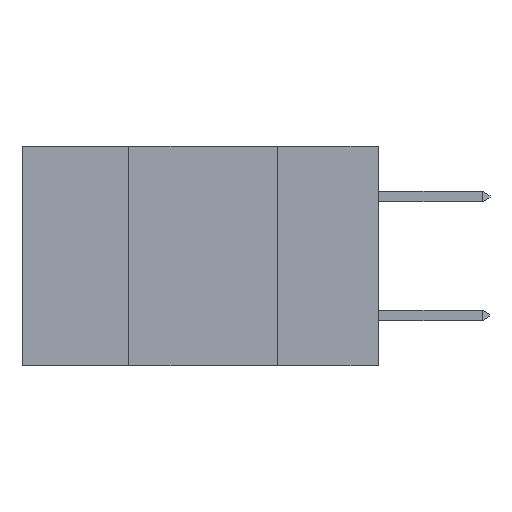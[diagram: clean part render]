
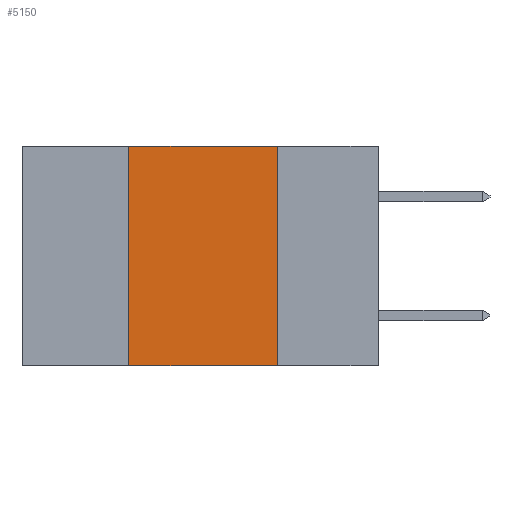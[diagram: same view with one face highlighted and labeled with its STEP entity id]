
A CAD part, left-side view. The second image highlights one B-rep face of the part: STEP entity #5150.
In plain terms, the highlighted planar face has unit normal (-1, 0, 0).
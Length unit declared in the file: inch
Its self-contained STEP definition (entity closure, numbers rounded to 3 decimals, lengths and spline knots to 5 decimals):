
#584 = ORIENTED_EDGE ( 'NONE', *, *, #10975, .F. ) ;
#1240 = VERTEX_POINT ( 'NONE', #1879 ) ;
#1879 = CARTESIAN_POINT ( 'NONE',  ( 0., 0.17, -0.37 ) ) ;
#2287 = DIRECTION ( 'NONE',  ( 0., 0., -1. ) ) ;
#2360 = VECTOR ( 'NONE', #20939, 39.37008 ) ;
#2624 = DIRECTION ( 'NONE',  ( 0., 0., 1. ) ) ;
#2678 = LINE ( 'NONE', #19572, #13314 ) ;
#2718 = ORIENTED_EDGE ( 'NONE', *, *, #19163, .F. ) ;
#2995 = CARTESIAN_POINT ( 'NONE',  ( 0., 0.42, -0.37 ) ) ;
#4079 = EDGE_CURVE ( 'NONE', #15891, #11140, #4483, .T. ) ;
#4483 = LINE ( 'NONE', #10596, #13944 ) ;
#5150 = ADVANCED_FACE ( 'NONE', ( #6834 ), #5991, .F. ) ;
#5981 = ORIENTED_EDGE ( 'NONE', *, *, #4079, .F. ) ;
#5991 = PLANE ( 'NONE',  #22442 ) ;
#6834 = FACE_OUTER_BOUND ( 'NONE', #9041, .T. ) ;
#7362 = LINE ( 'NONE', #9737, #2360 ) ;
#7534 = CARTESIAN_POINT ( 'NONE',  ( 0., 0.6, -0.37 ) ) ;
#9041 = EDGE_LOOP ( 'NONE', ( #584, #5981, #2718, #21029 ) ) ;
#9551 = LINE ( 'NONE', #7534, #15140 ) ;
#9737 = CARTESIAN_POINT ( 'NONE',  ( 0., 0.17, 0. ) ) ;
#10596 = CARTESIAN_POINT ( 'NONE',  ( 0., 0.6, 0. ) ) ;
#10975 = EDGE_CURVE ( 'NONE', #11140, #1240, #7362, .T. ) ;
#11140 = VERTEX_POINT ( 'NONE', #17555 ) ;
#12491 = DIRECTION ( 'NONE',  ( 0., -1., 0. ) ) ;
#13314 = VECTOR ( 'NONE', #2624, 39.37008 ) ;
#13595 = DIRECTION ( 'NONE',  ( 1., 0., 0. ) ) ;
#13944 = VECTOR ( 'NONE', #12491, 39.37008 ) ;
#15140 = VECTOR ( 'NONE', #20646, 39.37008 ) ;
#15447 = VERTEX_POINT ( 'NONE', #2995 ) ;
#15891 = VERTEX_POINT ( 'NONE', #19277 ) ;
#17555 = CARTESIAN_POINT ( 'NONE',  ( 0., 0.17, 0. ) ) ;
#19163 = EDGE_CURVE ( 'NONE', #15447, #15891, #2678, .T. ) ;
#19277 = CARTESIAN_POINT ( 'NONE',  ( 0., 0.42, 0. ) ) ;
#19572 = CARTESIAN_POINT ( 'NONE',  ( 0., 0.42, 0. ) ) ;
#20646 = DIRECTION ( 'NONE',  ( 0., -1., 0. ) ) ;
#20939 = DIRECTION ( 'NONE',  ( 0., 0., -1. ) ) ;
#21029 = ORIENTED_EDGE ( 'NONE', *, *, #22102, .T. ) ;
#22102 = EDGE_CURVE ( 'NONE', #15447, #1240, #9551, .T. ) ;
#22442 = AXIS2_PLACEMENT_3D ( 'NONE', #22894, #13595, #2287 ) ;
#22894 = CARTESIAN_POINT ( 'NONE',  ( 0., 0.6, 0. ) ) ;
